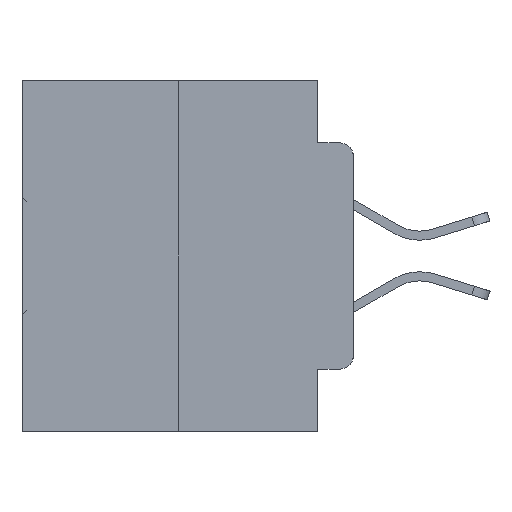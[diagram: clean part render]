
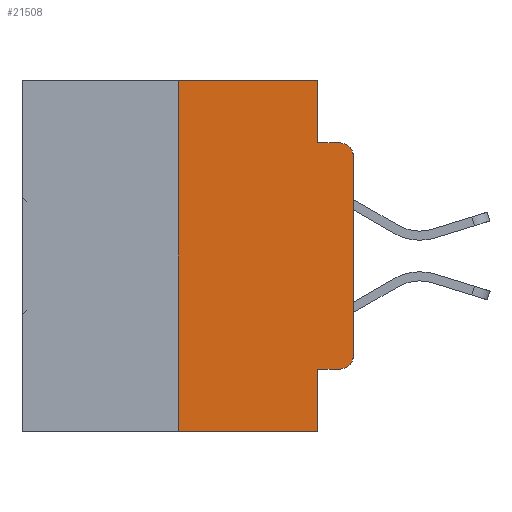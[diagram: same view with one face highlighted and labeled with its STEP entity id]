
A CAD part, left-side view. The second image highlights one B-rep face of the part: STEP entity #21508.
In plain terms, the highlighted planar face has unit normal (-1, 0, 0).
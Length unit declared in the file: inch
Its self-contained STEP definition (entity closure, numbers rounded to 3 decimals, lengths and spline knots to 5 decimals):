
#25 = EDGE_CURVE ( 'NONE', #22096, #33824, #15009, .T. ) ;
#30 = VERTEX_POINT ( 'NONE', #6719 ) ;
#497 = DIRECTION ( 'NONE',  ( 1., 0., 0. ) ) ;
#580 = DIRECTION ( 'NONE',  ( 0., -1., 0. ) ) ;
#688 = LINE ( 'NONE', #32397, #24884 ) ;
#931 = CARTESIAN_POINT ( 'NONE',  ( 0., 0.051, -0.4115 ) ) ;
#1204 = CIRCLE ( 'NONE', #18844, 0.02 ) ;
#1489 = DIRECTION ( 'NONE',  ( 0., -1., 0. ) ) ;
#1627 = LINE ( 'NONE', #4591, #2293 ) ;
#2050 = CARTESIAN_POINT ( 'NONE',  ( 0., 0., -0.1085 ) ) ;
#2154 = VERTEX_POINT ( 'NONE', #17682 ) ;
#2293 = VECTOR ( 'NONE', #15102, 39.37008 ) ;
#3549 = VECTOR ( 'NONE', #7627, 39.37008 ) ;
#3679 = CARTESIAN_POINT ( 'NONE',  ( 0., 0.02, -0.0885 ) ) ;
#4060 = ORIENTED_EDGE ( 'NONE', *, *, #29347, .F. ) ;
#4591 = CARTESIAN_POINT ( 'NONE',  ( 0., 0.25, 0. ) ) ;
#4874 = CARTESIAN_POINT ( 'NONE',  ( 0., 0.051, 0. ) ) ;
#5211 = LINE ( 'NONE', #4874, #3549 ) ;
#5701 = CIRCLE ( 'NONE', #15087, 0.02 ) ;
#6433 = CARTESIAN_POINT ( 'NONE',  ( 0., 0.25, 0. ) ) ;
#6719 = CARTESIAN_POINT ( 'NONE',  ( 0., 0.051, 0. ) ) ;
#7627 = DIRECTION ( 'NONE',  ( 0., 0., -1. ) ) ;
#7678 = VERTEX_POINT ( 'NONE', #3679 ) ;
#7702 = CARTESIAN_POINT ( 'NONE',  ( 0., 0.25, -0.5 ) ) ;
#8175 = EDGE_LOOP ( 'NONE', ( #22980, #22371, #30112, #9156, #4060, #12529, #18835, #20713, #26734, #12198 ) ) ;
#8651 = DIRECTION ( 'NONE',  ( 0., 0., -1. ) ) ;
#9112 = CARTESIAN_POINT ( 'NONE',  ( 0., 0., -0.3915 ) ) ;
#9156 = ORIENTED_EDGE ( 'NONE', *, *, #21341, .F. ) ;
#9318 = EDGE_CURVE ( 'NONE', #11828, #21768, #688, .T. ) ;
#9676 = VERTEX_POINT ( 'NONE', #32195 ) ;
#9727 = LINE ( 'NONE', #20210, #28319 ) ;
#10189 = EDGE_CURVE ( 'NONE', #30842, #21768, #29203, .T. ) ;
#11786 = CARTESIAN_POINT ( 'NONE',  ( 0., 0.051, -0.4115 ) ) ;
#11828 = VERTEX_POINT ( 'NONE', #11786 ) ;
#12198 = ORIENTED_EDGE ( 'NONE', *, *, #24335, .T. ) ;
#12529 = ORIENTED_EDGE ( 'NONE', *, *, #25873, .F. ) ;
#13779 = FACE_OUTER_BOUND ( 'NONE', #8175, .T. ) ;
#15009 = LINE ( 'NONE', #30667, #25588 ) ;
#15087 = AXIS2_PLACEMENT_3D ( 'NONE', #24184, #16623, #18883 ) ;
#15102 = DIRECTION ( 'NONE',  ( 0., 0., 1. ) ) ;
#15633 = VECTOR ( 'NONE', #29892, 39.37008 ) ;
#16623 = DIRECTION ( 'NONE',  ( -1., 0., 0. ) ) ;
#17013 = CARTESIAN_POINT ( 'NONE',  ( 0., 0.473, 0. ) ) ;
#17682 = CARTESIAN_POINT ( 'NONE',  ( 0., 0.02, -0.4115 ) ) ;
#18835 = ORIENTED_EDGE ( 'NONE', *, *, #10189, .T. ) ;
#18844 = AXIS2_PLACEMENT_3D ( 'NONE', #33987, #20565, #21064 ) ;
#18883 = DIRECTION ( 'NONE',  ( 0., 0., -1. ) ) ;
#19610 = LINE ( 'NONE', #17013, #26123 ) ;
#20210 = CARTESIAN_POINT ( 'NONE',  ( 0., 0.051, -0.0885 ) ) ;
#20329 = CARTESIAN_POINT ( 'NONE',  ( 0., 0.051, -0.5 ) ) ;
#20565 = DIRECTION ( 'NONE',  ( -1., 0., 0. ) ) ;
#20713 = ORIENTED_EDGE ( 'NONE', *, *, #9318, .F. ) ;
#21064 = DIRECTION ( 'NONE',  ( 0., 0., -1. ) ) ;
#21269 = EDGE_CURVE ( 'NONE', #9676, #7678, #9727, .T. ) ;
#21341 = EDGE_CURVE ( 'NONE', #30, #9676, #5211, .T. ) ;
#21508 = ADVANCED_FACE ( 'NONE', ( #13779 ), #31887, .F. ) ;
#21768 = VERTEX_POINT ( 'NONE', #20329 ) ;
#21957 = LINE ( 'NONE', #931, #15633 ) ;
#22096 = VERTEX_POINT ( 'NONE', #9112 ) ;
#22371 = ORIENTED_EDGE ( 'NONE', *, *, #27874, .T. ) ;
#22980 = ORIENTED_EDGE ( 'NONE', *, *, #25, .T. ) ;
#23978 = VERTEX_POINT ( 'NONE', #6433 ) ;
#24184 = CARTESIAN_POINT ( 'NONE',  ( 0., 0.02, -0.1085 ) ) ;
#24335 = EDGE_CURVE ( 'NONE', #2154, #22096, #1204, .T. ) ;
#24370 = VECTOR ( 'NONE', #580, 39.37008 ) ;
#24884 = VECTOR ( 'NONE', #8651, 39.37008 ) ;
#25588 = VECTOR ( 'NONE', #30493, 39.37008 ) ;
#25873 = EDGE_CURVE ( 'NONE', #30842, #23978, #1627, .T. ) ;
#26123 = VECTOR ( 'NONE', #1489, 39.37008 ) ;
#26734 = ORIENTED_EDGE ( 'NONE', *, *, #31095, .T. ) ;
#27874 = EDGE_CURVE ( 'NONE', #33824, #7678, #5701, .T. ) ;
#28319 = VECTOR ( 'NONE', #28968, 39.37008 ) ;
#28968 = DIRECTION ( 'NONE',  ( 0., -1., 0. ) ) ;
#29203 = LINE ( 'NONE', #32143, #24370 ) ;
#29284 = DIRECTION ( 'NONE',  ( 0., 0., -1. ) ) ;
#29347 = EDGE_CURVE ( 'NONE', #23978, #30, #19610, .T. ) ;
#29892 = DIRECTION ( 'NONE',  ( 0., -1., 0. ) ) ;
#30112 = ORIENTED_EDGE ( 'NONE', *, *, #21269, .F. ) ;
#30493 = DIRECTION ( 'NONE',  ( 0., 0., 1. ) ) ;
#30667 = CARTESIAN_POINT ( 'NONE',  ( 0., 0., 0. ) ) ;
#30842 = VERTEX_POINT ( 'NONE', #7702 ) ;
#31080 = AXIS2_PLACEMENT_3D ( 'NONE', #32233, #497, #29284 ) ;
#31095 = EDGE_CURVE ( 'NONE', #11828, #2154, #21957, .T. ) ;
#31887 = PLANE ( 'NONE',  #31080 ) ;
#32143 = CARTESIAN_POINT ( 'NONE',  ( 0., 0.473, -0.5 ) ) ;
#32195 = CARTESIAN_POINT ( 'NONE',  ( 0., 0.051, -0.0885 ) ) ;
#32233 = CARTESIAN_POINT ( 'NONE',  ( 0., 0.473, 0. ) ) ;
#32397 = CARTESIAN_POINT ( 'NONE',  ( 0., 0.051, 0. ) ) ;
#33824 = VERTEX_POINT ( 'NONE', #2050 ) ;
#33987 = CARTESIAN_POINT ( 'NONE',  ( 0., 0.02, -0.3915 ) ) ;
